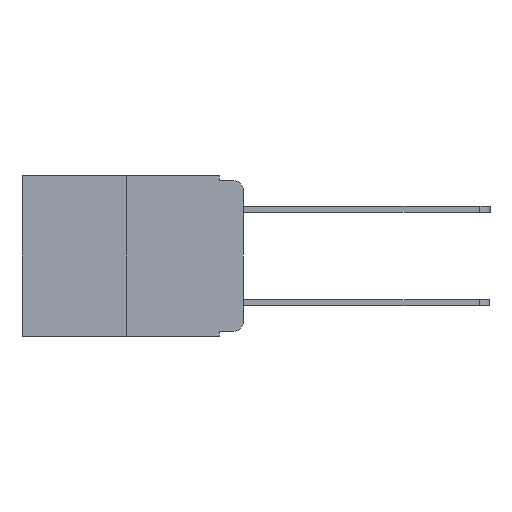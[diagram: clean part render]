
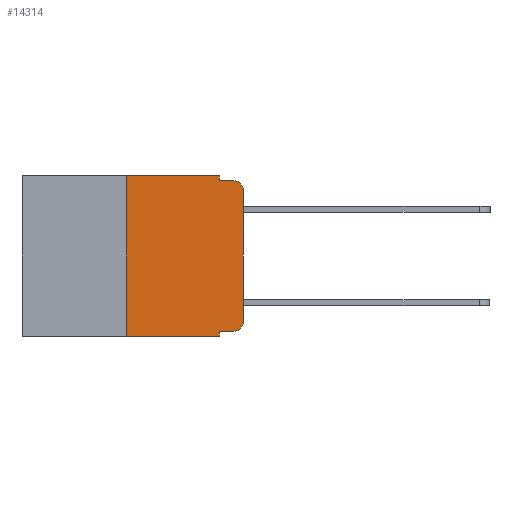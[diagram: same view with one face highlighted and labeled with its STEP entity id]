
A CAD part, left-side view. The second image highlights one B-rep face of the part: STEP entity #14314.
In plain terms, the highlighted planar face has unit normal (-1, 0, 0).
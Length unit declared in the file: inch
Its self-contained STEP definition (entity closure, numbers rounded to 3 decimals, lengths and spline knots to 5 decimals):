
#832 = DIRECTION ( 'NONE',  ( 0., 0., -1. ) ) ;
#850 = DIRECTION ( 'NONE',  ( 0., 0., -1. ) ) ;
#1350 = VERTEX_POINT ( 'NONE', #7911 ) ;
#1519 = ORIENTED_EDGE ( 'NONE', *, *, #14751, .T. ) ;
#2278 = CARTESIAN_POINT ( 'NONE',  ( 0., 0.25, 0. ) ) ;
#2553 = EDGE_CURVE ( 'NONE', #6956, #3117, #6649, .T. ) ;
#3117 = VERTEX_POINT ( 'NONE', #19812 ) ;
#3359 = LINE ( 'NONE', #11722, #15017 ) ;
#3715 = CIRCLE ( 'NONE', #17243, 0.02 ) ;
#3763 = EDGE_CURVE ( 'NONE', #1350, #9733, #18878, .T. ) ;
#3789 = CARTESIAN_POINT ( 'NONE',  ( 0., 0.02, -0.333 ) ) ;
#4079 = LINE ( 'NONE', #12399, #15647 ) ;
#4118 = DIRECTION ( 'NONE',  ( 0., 0., 1. ) ) ;
#4216 = CARTESIAN_POINT ( 'NONE',  ( 0., 0.051, -0.333 ) ) ;
#4397 = CARTESIAN_POINT ( 'NONE',  ( 0., 0.051, -0.343 ) ) ;
#4623 = VECTOR ( 'NONE', #5502, 39.37008 ) ;
#5044 = ORIENTED_EDGE ( 'NONE', *, *, #17786, .F. ) ;
#5063 = CARTESIAN_POINT ( 'NONE',  ( 0., 0., -0.03 ) ) ;
#5502 = DIRECTION ( 'NONE',  ( 0., -1., 0. ) ) ;
#5922 = CARTESIAN_POINT ( 'NONE',  ( 0., 0.051, 0. ) ) ;
#6152 = VECTOR ( 'NONE', #19889, 39.37008 ) ;
#6649 = LINE ( 'NONE', #5922, #6152 ) ;
#6956 = VERTEX_POINT ( 'NONE', #13414 ) ;
#7268 = LINE ( 'NONE', #10570, #12456 ) ;
#7633 = PLANE ( 'NONE',  #11729 ) ;
#7732 = DIRECTION ( 'NONE',  ( -1., 0., 0. ) ) ;
#7812 = VERTEX_POINT ( 'NONE', #19309 ) ;
#7911 = CARTESIAN_POINT ( 'NONE',  ( 0., 0.25, -0.343 ) ) ;
#8036 = EDGE_CURVE ( 'NONE', #19927, #10005, #4079, .T. ) ;
#8038 = VECTOR ( 'NONE', #16313, 39.37008 ) ;
#8744 = DIRECTION ( 'NONE',  ( 0., -1., 0. ) ) ;
#8905 = FACE_OUTER_BOUND ( 'NONE', #20144, .T. ) ;
#9105 = EDGE_CURVE ( 'NONE', #19927, #17794, #9367, .T. ) ;
#9367 = LINE ( 'NONE', #4216, #4623 ) ;
#9395 = CARTESIAN_POINT ( 'NONE',  ( 0., 0.02, -0.313 ) ) ;
#9733 = VERTEX_POINT ( 'NONE', #12601 ) ;
#10005 = VERTEX_POINT ( 'NONE', #4397 ) ;
#10570 = CARTESIAN_POINT ( 'NONE',  ( 0., 0.051, -0.01 ) ) ;
#10696 = VECTOR ( 'NONE', #4118, 39.37008 ) ;
#10839 = DIRECTION ( 'NONE',  ( 1., 0., 0. ) ) ;
#11009 = DIRECTION ( 'NONE',  ( 0., 0., -1. ) ) ;
#11037 = CIRCLE ( 'NONE', #12184, 0.02 ) ;
#11044 = ORIENTED_EDGE ( 'NONE', *, *, #12295, .T. ) ;
#11489 = EDGE_CURVE ( 'NONE', #1350, #10005, #13432, .T. ) ;
#11722 = CARTESIAN_POINT ( 'NONE',  ( 0., 0., 0. ) ) ;
#11729 = AXIS2_PLACEMENT_3D ( 'NONE', #20024, #10839, #850 ) ;
#11761 = ORIENTED_EDGE ( 'NONE', *, *, #2553, .F. ) ;
#12002 = ORIENTED_EDGE ( 'NONE', *, *, #8036, .F. ) ;
#12134 = DIRECTION ( 'NONE',  ( 0., -1., 0. ) ) ;
#12184 = AXIS2_PLACEMENT_3D ( 'NONE', #17062, #7732, #18595 ) ;
#12295 = EDGE_CURVE ( 'NONE', #17794, #13100, #3715, .T. ) ;
#12399 = CARTESIAN_POINT ( 'NONE',  ( 0., 0.051, 0. ) ) ;
#12456 = VECTOR ( 'NONE', #12134, 39.37008 ) ;
#12601 = CARTESIAN_POINT ( 'NONE',  ( 0., 0.25, 0. ) ) ;
#12930 = VECTOR ( 'NONE', #8744, 39.37008 ) ;
#13100 = VERTEX_POINT ( 'NONE', #14217 ) ;
#13414 = CARTESIAN_POINT ( 'NONE',  ( 0., 0.051, 0. ) ) ;
#13432 = LINE ( 'NONE', #14969, #12930 ) ;
#14217 = CARTESIAN_POINT ( 'NONE',  ( 0., 0., -0.313 ) ) ;
#14314 = ADVANCED_FACE ( 'NONE', ( #8905 ), #7633, .F. ) ;
#14751 = EDGE_CURVE ( 'NONE', #13100, #17665, #3359, .T. ) ;
#14773 = CARTESIAN_POINT ( 'NONE',  ( 0., 0.473, 0. ) ) ;
#14969 = CARTESIAN_POINT ( 'NONE',  ( 0., 0.473, -0.343 ) ) ;
#15017 = VECTOR ( 'NONE', #16370, 39.37008 ) ;
#15647 = VECTOR ( 'NONE', #832, 39.37008 ) ;
#16088 = ORIENTED_EDGE ( 'NONE', *, *, #19847, .F. ) ;
#16313 = DIRECTION ( 'NONE',  ( 0., -1., 0. ) ) ;
#16370 = DIRECTION ( 'NONE',  ( 0., 0., 1. ) ) ;
#17062 = CARTESIAN_POINT ( 'NONE',  ( 0., 0.02, -0.03 ) ) ;
#17243 = AXIS2_PLACEMENT_3D ( 'NONE', #9395, #20168, #11009 ) ;
#17514 = ORIENTED_EDGE ( 'NONE', *, *, #11489, .T. ) ;
#17665 = VERTEX_POINT ( 'NONE', #5063 ) ;
#17786 = EDGE_CURVE ( 'NONE', #9733, #6956, #20359, .T. ) ;
#17794 = VERTEX_POINT ( 'NONE', #3789 ) ;
#18007 = ORIENTED_EDGE ( 'NONE', *, *, #9105, .T. ) ;
#18499 = CARTESIAN_POINT ( 'NONE',  ( 0., 0.051, -0.333 ) ) ;
#18595 = DIRECTION ( 'NONE',  ( 0., 0., -1. ) ) ;
#18727 = ORIENTED_EDGE ( 'NONE', *, *, #18834, .T. ) ;
#18834 = EDGE_CURVE ( 'NONE', #17665, #7812, #11037, .T. ) ;
#18878 = LINE ( 'NONE', #2278, #10696 ) ;
#19309 = CARTESIAN_POINT ( 'NONE',  ( 0., 0.02, -0.01 ) ) ;
#19812 = CARTESIAN_POINT ( 'NONE',  ( 0., 0.051, -0.01 ) ) ;
#19847 = EDGE_CURVE ( 'NONE', #3117, #7812, #7268, .T. ) ;
#19889 = DIRECTION ( 'NONE',  ( 0., 0., -1. ) ) ;
#19927 = VERTEX_POINT ( 'NONE', #18499 ) ;
#20024 = CARTESIAN_POINT ( 'NONE',  ( 0., 0.473, 0. ) ) ;
#20144 = EDGE_LOOP ( 'NONE', ( #1519, #18727, #16088, #11761, #5044, #20583, #17514, #12002, #18007, #11044 ) ) ;
#20168 = DIRECTION ( 'NONE',  ( -1., 0., 0. ) ) ;
#20359 = LINE ( 'NONE', #14773, #8038 ) ;
#20583 = ORIENTED_EDGE ( 'NONE', *, *, #3763, .F. ) ;
